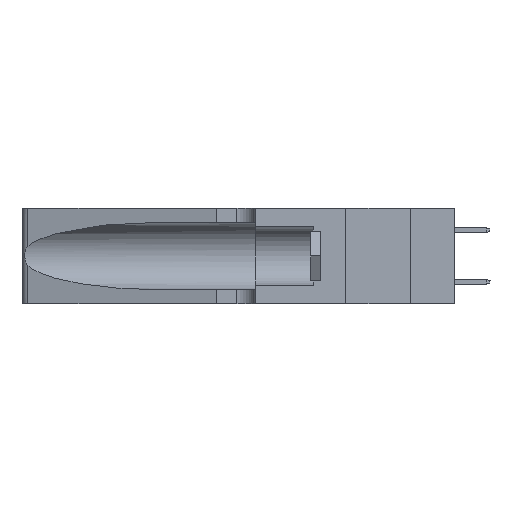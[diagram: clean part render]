
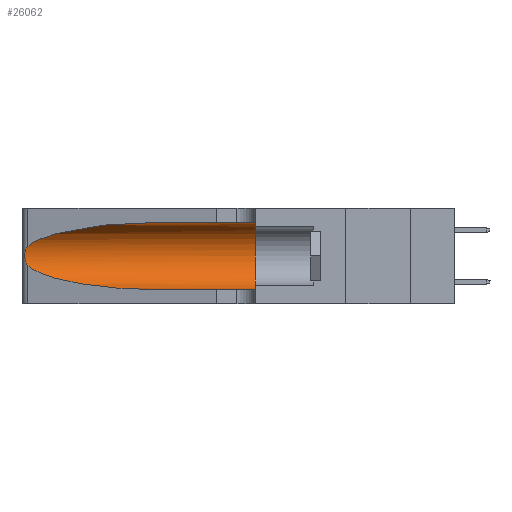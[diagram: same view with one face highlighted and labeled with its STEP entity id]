
A CAD part, left-side view. The second image highlights one B-rep face of the part: STEP entity #26062.
In plain terms, the highlighted cylindrical face has radius 3.308 mm (diameter 6.617 mm), a partial arc.
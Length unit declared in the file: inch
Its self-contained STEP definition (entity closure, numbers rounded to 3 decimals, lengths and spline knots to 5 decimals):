
#1227 = CARTESIAN_POINT ( 'NONE',  ( 0.18966, 0.96281, 0.05475 ) ) ;
#2312 = CARTESIAN_POINT ( 'NONE',  ( 0.26075, 1.23896, 0.19203 ) ) ;
#2811 = AXIS2_PLACEMENT_3D ( 'NONE', #41368, #25924, #8947 ) ;
#2913 = EDGE_CURVE ( 'NONE', #29237, #34968, #35112, .T. ) ;
#5249 = ORIENTED_EDGE ( 'NONE', *, *, #21405, .F. ) ;
#5299 = CARTESIAN_POINT ( 'NONE',  ( 0.25487, 1.22718, 0.14631 ) ) ;
#6411 = EDGE_LOOP ( 'NONE', ( #41773, #12007, #8018, #7128, #7253, #5249 ) ) ;
#6691 = EDGE_CURVE ( 'NONE', #17055, #12614, #17731, .T. ) ;
#7128 = ORIENTED_EDGE ( 'NONE', *, *, #20864, .T. ) ;
#7179 = DIRECTION ( 'NONE',  ( 0., 0., 1. ) ) ;
#7253 = ORIENTED_EDGE ( 'NONE', *, *, #2913, .F. ) ;
#8018 = ORIENTED_EDGE ( 'NONE', *, *, #15919, .T. ) ;
#8044 = CARTESIAN_POINT ( 'NONE',  ( 0.25487, 1.22718, 0.14631 ) ) ;
#8475 = CARTESIAN_POINT ( 'NONE',  ( 0.25639, 1.23186, 0.15144 ) ) ;
#8947 = DIRECTION ( 'NONE',  ( 0., 0., -1. ) ) ;
#9306 = CARTESIAN_POINT ( 'NONE',  ( 0.26018, 1.23835, 0.19895 ) ) ;
#9610 = CARTESIAN_POINT ( 'NONE',  ( 0.25487, 1.22718, 0.22369 ) ) ;
#10656 = DIRECTION ( 'NONE',  ( 0., -1., 0. ) ) ;
#11107 = VERTEX_POINT ( 'NONE', #11409 ) ;
#11409 = CARTESIAN_POINT ( 'NONE',  ( 0.1305, 0.72297, 0.05475 ) ) ;
#11676 = CARTESIAN_POINT ( 'NONE',  ( 0.26075, 1.23896, 0.178 ) ) ;
#12007 = ORIENTED_EDGE ( 'NONE', *, *, #40783, .T. ) ;
#12489 = CARTESIAN_POINT ( 'NONE',  ( 0.25555, 1.22994, 0.2215 ) ) ;
#12614 = VERTEX_POINT ( 'NONE', #15248 ) ;
#13157 = B_SPLINE_CURVE_WITH_KNOTS ( 'NONE', 3,
 ( #15265, #12489, #31372, #25440, #25034, #9306, #2312, #11676, #37888, #24618, #37477, #8475, #21474, #5299 ),
 .UNSPECIFIED., .F., .F.,
 ( 4, 2, 2, 2, 2, 2, 4 ),
 ( 0., 0.00027, 0.00053, 0.00107, 0.0016, 0.00187, 0.00214 ),
 .UNSPECIFIED. ) ;
#13615 = LINE ( 'NONE', #36692, #34347 ) ;
#13719 = CARTESIAN_POINT ( 'NONE',  ( 0.2373, 1.15595, 0.08982 ) ) ;
#15248 = CARTESIAN_POINT ( 'NONE',  ( 0.25487, 1.22718, 0.22369 ) ) ;
#15265 = CARTESIAN_POINT ( 'NONE',  ( 0.25487, 1.22718, 0.22369 ) ) ;
#15408 = VECTOR ( 'NONE', #36656, 39.37008 ) ;
#15919 = EDGE_CURVE ( 'NONE', #23748, #11107, #36104, .T. ) ;
#15978 = CYLINDRICAL_SURFACE ( 'NONE', #2811, 0.13025 ) ;
#17055 = VERTEX_POINT ( 'NONE', #24437 ) ;
#17142 = CARTESIAN_POINT ( 'NONE',  ( 0.1305, 0.72297, 0.05475 ) ) ;
#17731 =( BOUNDED_CURVE ( )  B_SPLINE_CURVE ( 3, ( #41182, #22584, #25750, #9610 ),
 .UNSPECIFIED., .F., .F. ) 
 B_SPLINE_CURVE_WITH_KNOTS ( ( 4, 4 ),
 ( 1.5708, 2.84003 ),
 .UNSPECIFIED. ) 
 CURVE ( )  GEOMETRIC_REPRESENTATION_ITEM ( )  RATIONAL_B_SPLINE_CURVE ( ( 1., 0.87, 0.87, 1. ) ) 
 REPRESENTATION_ITEM ( '' )  );
#19671 = CARTESIAN_POINT ( 'NONE',  ( 0.1305, 0.35, 0.31525 ) ) ;
#20393 = LINE ( 'NONE', #33268, #15408 ) ;
#20864 = EDGE_CURVE ( 'NONE', #11107, #34968, #13615, .T. ) ;
#21405 = EDGE_CURVE ( 'NONE', #17055, #29237, #20393, .T. ) ;
#21474 = CARTESIAN_POINT ( 'NONE',  ( 0.25555, 1.22993, 0.14849 ) ) ;
#22584 = CARTESIAN_POINT ( 'NONE',  ( 0.18966, 0.96281, 0.31525 ) ) ;
#23748 = VERTEX_POINT ( 'NONE', #8044 ) ;
#24437 = CARTESIAN_POINT ( 'NONE',  ( 0.1305, 0.72297, 0.31525 ) ) ;
#24618 = CARTESIAN_POINT ( 'NONE',  ( 0.25856, 1.23593, 0.16098 ) ) ;
#25034 = CARTESIAN_POINT ( 'NONE',  ( 0.25854, 1.2359, 0.20912 ) ) ;
#25440 = CARTESIAN_POINT ( 'NONE',  ( 0.25787, 1.23484, 0.2124 ) ) ;
#25750 = CARTESIAN_POINT ( 'NONE',  ( 0.2373, 1.15595, 0.28018 ) ) ;
#25924 = DIRECTION ( 'NONE',  ( 0., -1., 0. ) ) ;
#26062 = ADVANCED_FACE ( 'NONE', ( #38796 ), #15978, .F. ) ;
#28786 = DIRECTION ( 'NONE',  ( 0., 1., 0. ) ) ;
#29237 = VERTEX_POINT ( 'NONE', #19671 ) ;
#31067 = AXIS2_PLACEMENT_3D ( 'NONE', #32164, #28786, #7179 ) ;
#31372 = CARTESIAN_POINT ( 'NONE',  ( 0.25639, 1.23184, 0.21858 ) ) ;
#32164 = CARTESIAN_POINT ( 'NONE',  ( 0.1305, 0.35, 0.185 ) ) ;
#33268 = CARTESIAN_POINT ( 'NONE',  ( 0.1305, 1.61858, 0.31525 ) ) ;
#34347 = VECTOR ( 'NONE', #10656, 39.37008 ) ;
#34968 = VERTEX_POINT ( 'NONE', #40980 ) ;
#35112 = CIRCLE ( 'NONE', #31067, 0.13025 ) ;
#36104 =( BOUNDED_CURVE ( )  B_SPLINE_CURVE ( 3, ( #36385, #13719, #1227, #17142 ),
 .UNSPECIFIED., .F., .T. ) 
 B_SPLINE_CURVE_WITH_KNOTS ( ( 4, 4 ),
 ( 3.44316, 4.71239 ),
 .UNSPECIFIED. ) 
 CURVE ( )  GEOMETRIC_REPRESENTATION_ITEM ( )  RATIONAL_B_SPLINE_CURVE ( ( 1., 0.87, 0.87, 1. ) ) 
 REPRESENTATION_ITEM ( '' )  );
#36385 = CARTESIAN_POINT ( 'NONE',  ( 0.25487, 1.22718, 0.14631 ) ) ;
#36656 = DIRECTION ( 'NONE',  ( 0., -1., 0. ) ) ;
#36692 = CARTESIAN_POINT ( 'NONE',  ( 0.1305, 1.61858, 0.05475 ) ) ;
#37477 = CARTESIAN_POINT ( 'NONE',  ( 0.25789, 1.23486, 0.15765 ) ) ;
#37888 = CARTESIAN_POINT ( 'NONE',  ( 0.26017, 1.23833, 0.17102 ) ) ;
#38796 = FACE_OUTER_BOUND ( 'NONE', #6411, .T. ) ;
#40783 = EDGE_CURVE ( 'NONE', #12614, #23748, #13157, .T. ) ;
#40980 = CARTESIAN_POINT ( 'NONE',  ( 0.1305, 0.35, 0.05475 ) ) ;
#41182 = CARTESIAN_POINT ( 'NONE',  ( 0.1305, 0.72297, 0.31525 ) ) ;
#41368 = CARTESIAN_POINT ( 'NONE',  ( 0.1305, 1.61858, 0.185 ) ) ;
#41773 = ORIENTED_EDGE ( 'NONE', *, *, #6691, .T. ) ;
